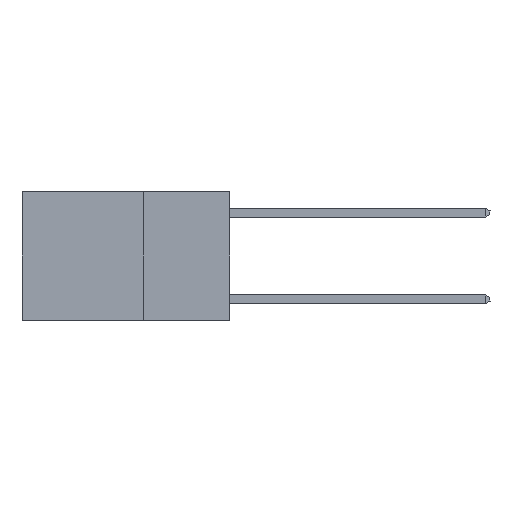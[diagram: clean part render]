
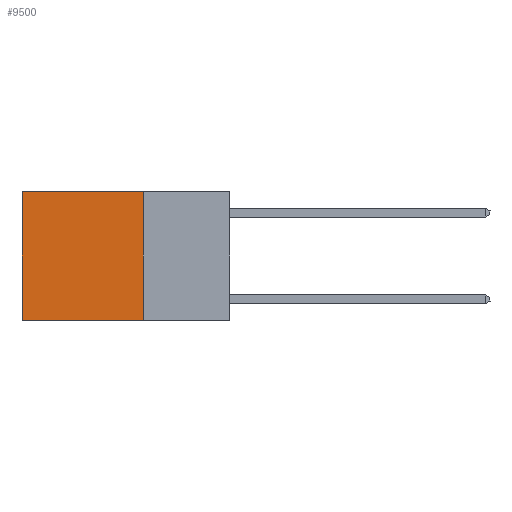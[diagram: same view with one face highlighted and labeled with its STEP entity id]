
A CAD part, left-side view. The second image highlights one B-rep face of the part: STEP entity #9500.
In plain terms, the highlighted planar face has unit normal (-1, 0, 0).
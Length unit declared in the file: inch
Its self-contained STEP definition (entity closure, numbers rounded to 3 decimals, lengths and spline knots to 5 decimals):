
#126 = VERTEX_POINT ( 'NONE', #2645 ) ;
#179 = VECTOR ( 'NONE', #12389, 39.37008 ) ;
#788 = LINE ( 'NONE', #25583, #179 ) ;
#2238 = ORIENTED_EDGE ( 'NONE', *, *, #12699, .T. ) ;
#2645 = CARTESIAN_POINT ( 'NONE',  ( 0.2625, 0.6, -0.37 ) ) ;
#3569 = CARTESIAN_POINT ( 'NONE',  ( 0.2625, 0.6, 0. ) ) ;
#4659 = VERTEX_POINT ( 'NONE', #6337 ) ;
#4806 = CARTESIAN_POINT ( 'NONE',  ( 0.2625, 0.25, 0. ) ) ;
#5816 = ORIENTED_EDGE ( 'NONE', *, *, #15993, .F. ) ;
#6337 = CARTESIAN_POINT ( 'NONE',  ( 0.2625, 0.25, 0. ) ) ;
#7806 = ORIENTED_EDGE ( 'NONE', *, *, #26535, .F. ) ;
#9500 = ADVANCED_FACE ( 'NONE', ( #14293 ), #27660, .F. ) ;
#9670 = LINE ( 'NONE', #3569, #22292 ) ;
#9843 = VERTEX_POINT ( 'NONE', #20906 ) ;
#10081 = DIRECTION ( 'NONE',  ( 0., 1., 0. ) ) ;
#11022 = VECTOR ( 'NONE', #10081, 39.37008 ) ;
#12167 = EDGE_LOOP ( 'NONE', ( #2238, #7806, #5816, #23074 ) ) ;
#12259 = LINE ( 'NONE', #21097, #11022 ) ;
#12389 = DIRECTION ( 'NONE',  ( 0., 0., -1. ) ) ;
#12699 = EDGE_CURVE ( 'NONE', #9843, #126, #9670, .T. ) ;
#14293 = FACE_OUTER_BOUND ( 'NONE', #12167, .T. ) ;
#15993 = EDGE_CURVE ( 'NONE', #4659, #24876, #788, .T. ) ;
#16777 = DIRECTION ( 'NONE',  ( 0., 1., 0. ) ) ;
#18786 = VECTOR ( 'NONE', #16777, 39.37008 ) ;
#20407 = EDGE_CURVE ( 'NONE', #4659, #9843, #21912, .T. ) ;
#20906 = CARTESIAN_POINT ( 'NONE',  ( 0.2625, 0.6, 0. ) ) ;
#21097 = CARTESIAN_POINT ( 'NONE',  ( 0.2625, 0.25, -0.37 ) ) ;
#21871 = CARTESIAN_POINT ( 'NONE',  ( 0.2625, 0.25, -0.37 ) ) ;
#21912 = LINE ( 'NONE', #4806, #18786 ) ;
#22292 = VECTOR ( 'NONE', #25031, 39.37008 ) ;
#23074 = ORIENTED_EDGE ( 'NONE', *, *, #20407, .T. ) ;
#23151 = CARTESIAN_POINT ( 'NONE',  ( 0.2625, 0.25, 0. ) ) ;
#23588 = AXIS2_PLACEMENT_3D ( 'NONE', #23151, #27092, #27230 ) ;
#24876 = VERTEX_POINT ( 'NONE', #21871 ) ;
#25031 = DIRECTION ( 'NONE',  ( 0., 0., -1. ) ) ;
#25583 = CARTESIAN_POINT ( 'NONE',  ( 0.2625, 0.25, 0. ) ) ;
#26535 = EDGE_CURVE ( 'NONE', #24876, #126, #12259, .T. ) ;
#27092 = DIRECTION ( 'NONE',  ( 1., 0., 0. ) ) ;
#27230 = DIRECTION ( 'NONE',  ( 0., 0., -1. ) ) ;
#27660 = PLANE ( 'NONE',  #23588 ) ;
